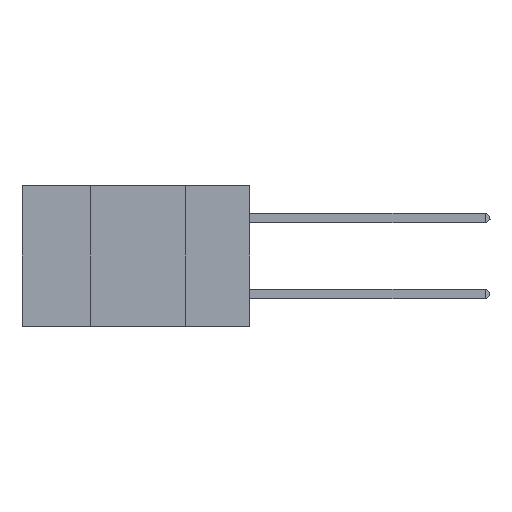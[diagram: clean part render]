
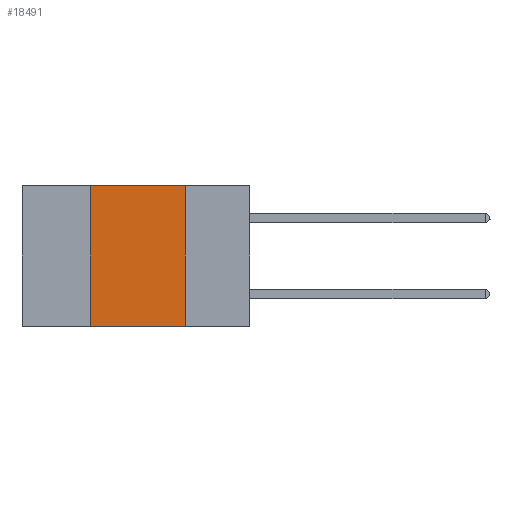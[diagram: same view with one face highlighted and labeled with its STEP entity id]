
A CAD part, left-side view. The second image highlights one B-rep face of the part: STEP entity #18491.
In plain terms, the highlighted planar face has unit normal (-1, 0, 0).
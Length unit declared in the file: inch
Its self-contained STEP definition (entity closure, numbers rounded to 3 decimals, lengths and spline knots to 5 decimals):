
#409 = VECTOR ( 'NONE', #2832, 39.37008 ) ;
#1203 = CARTESIAN_POINT ( 'NONE',  ( 0., 0.42, 0. ) ) ;
#2202 = PLANE ( 'NONE',  #18212 ) ;
#2298 = FACE_OUTER_BOUND ( 'NONE', #10818, .T. ) ;
#2832 = DIRECTION ( 'NONE',  ( 0., 0., 1. ) ) ;
#3137 = ORIENTED_EDGE ( 'NONE', *, *, #17150, .F. ) ;
#3143 = CARTESIAN_POINT ( 'NONE',  ( 0., 0.6, -0.37 ) ) ;
#3977 = ORIENTED_EDGE ( 'NONE', *, *, #7345, .F. ) ;
#4439 = DIRECTION ( 'NONE',  ( 0., -1., 0. ) ) ;
#4869 = EDGE_CURVE ( 'NONE', #11856, #17280, #12572, .T. ) ;
#6684 = VERTEX_POINT ( 'NONE', #1203 ) ;
#7345 = EDGE_CURVE ( 'NONE', #9079, #6684, #11392, .T. ) ;
#7762 = CARTESIAN_POINT ( 'NONE',  ( 0., 0.17, 0. ) ) ;
#8831 = CARTESIAN_POINT ( 'NONE',  ( 0., 0.6, 0. ) ) ;
#9079 = VERTEX_POINT ( 'NONE', #17362 ) ;
#9271 = CARTESIAN_POINT ( 'NONE',  ( 0., 0.17, 0. ) ) ;
#10347 = LINE ( 'NONE', #16574, #14041 ) ;
#10756 = ORIENTED_EDGE ( 'NONE', *, *, #13850, .T. ) ;
#10818 = EDGE_LOOP ( 'NONE', ( #14796, #3137, #3977, #10756 ) ) ;
#11392 = LINE ( 'NONE', #12888, #409 ) ;
#11856 = VERTEX_POINT ( 'NONE', #9271 ) ;
#12572 = LINE ( 'NONE', #7762, #20215 ) ;
#12883 = LINE ( 'NONE', #3143, #18072 ) ;
#12888 = CARTESIAN_POINT ( 'NONE',  ( 0., 0.42, 0. ) ) ;
#13249 = DIRECTION ( 'NONE',  ( 0., -1., 0. ) ) ;
#13850 = EDGE_CURVE ( 'NONE', #9079, #17280, #12883, .T. ) ;
#14041 = VECTOR ( 'NONE', #13249, 39.37008 ) ;
#14796 = ORIENTED_EDGE ( 'NONE', *, *, #4869, .F. ) ;
#15363 = DIRECTION ( 'NONE',  ( 1., 0., 0. ) ) ;
#15680 = DIRECTION ( 'NONE',  ( 0., 0., -1. ) ) ;
#16574 = CARTESIAN_POINT ( 'NONE',  ( 0., 0.6, 0. ) ) ;
#17150 = EDGE_CURVE ( 'NONE', #6684, #11856, #10347, .T. ) ;
#17280 = VERTEX_POINT ( 'NONE', #18797 ) ;
#17362 = CARTESIAN_POINT ( 'NONE',  ( 0., 0.42, -0.37 ) ) ;
#18072 = VECTOR ( 'NONE', #4439, 39.37008 ) ;
#18212 = AXIS2_PLACEMENT_3D ( 'NONE', #8831, #15363, #19894 ) ;
#18491 = ADVANCED_FACE ( 'NONE', ( #2298 ), #2202, .F. ) ;
#18797 = CARTESIAN_POINT ( 'NONE',  ( 0., 0.17, -0.37 ) ) ;
#19894 = DIRECTION ( 'NONE',  ( 0., 0., -1. ) ) ;
#20215 = VECTOR ( 'NONE', #15680, 39.37008 ) ;
